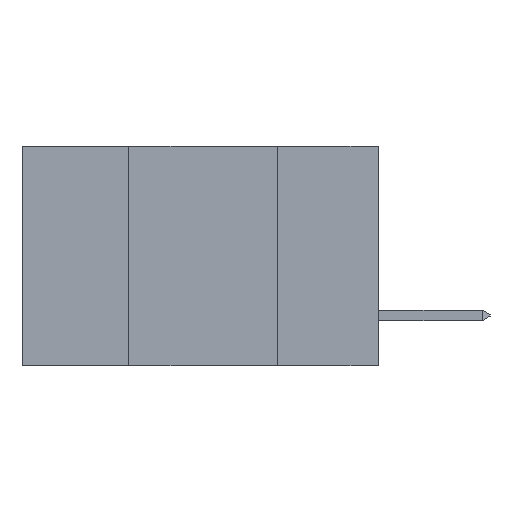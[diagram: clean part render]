
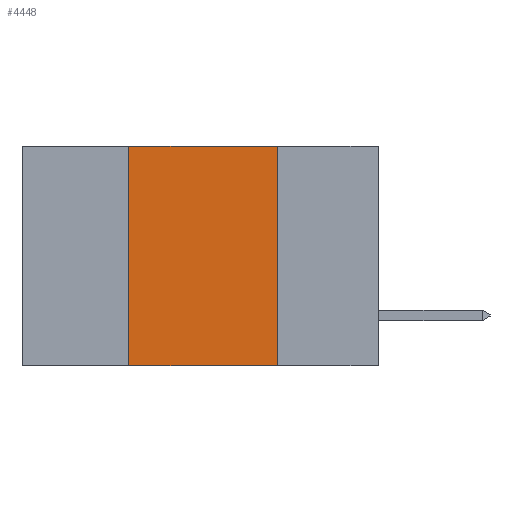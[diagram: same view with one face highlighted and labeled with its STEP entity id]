
A CAD part, left-side view. The second image highlights one B-rep face of the part: STEP entity #4448.
In plain terms, the highlighted planar face has unit normal (-1, 0, 0).
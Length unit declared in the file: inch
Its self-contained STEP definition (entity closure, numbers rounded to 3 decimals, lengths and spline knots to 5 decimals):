
#2800 = VERTEX_POINT ( 'NONE', #9452 ) ;
#3032 = DIRECTION ( 'NONE',  ( 0., 0., -1. ) ) ;
#3098 = DIRECTION ( 'NONE',  ( 1., 0., 0. ) ) ;
#4194 = VECTOR ( 'NONE', #26800, 39.37008 ) ;
#4448 = ADVANCED_FACE ( 'NONE', ( #22939 ), #6076, .F. ) ;
#4514 = CARTESIAN_POINT ( 'NONE',  ( 0., 0.17, 0. ) ) ;
#4547 = EDGE_CURVE ( 'NONE', #25164, #24724, #20202, .T. ) ;
#5257 = CARTESIAN_POINT ( 'NONE',  ( 0., 0.6, 0. ) ) ;
#6076 = PLANE ( 'NONE',  #16238 ) ;
#9062 = CARTESIAN_POINT ( 'NONE',  ( 0., 0.6, -0.37 ) ) ;
#9239 = EDGE_LOOP ( 'NONE', ( #10128, #17711, #11962, #24147 ) ) ;
#9452 = CARTESIAN_POINT ( 'NONE',  ( 0., 0.42, 0. ) ) ;
#9957 = VECTOR ( 'NONE', #14815, 39.37008 ) ;
#10106 = EDGE_CURVE ( 'NONE', #20956, #24724, #22826, .T. ) ;
#10128 = ORIENTED_EDGE ( 'NONE', *, *, #4547, .F. ) ;
#11547 = CARTESIAN_POINT ( 'NONE',  ( 0., 0.42, -0.37 ) ) ;
#11705 = EDGE_CURVE ( 'NONE', #2800, #25164, #14842, .T. ) ;
#11962 = ORIENTED_EDGE ( 'NONE', *, *, #20606, .F. ) ;
#12812 = CARTESIAN_POINT ( 'NONE',  ( 0., 0.42, 0. ) ) ;
#13532 = VECTOR ( 'NONE', #24804, 39.37008 ) ;
#14151 = CARTESIAN_POINT ( 'NONE',  ( 0., 0.6, 0. ) ) ;
#14815 = DIRECTION ( 'NONE',  ( 0., 0., 1. ) ) ;
#14842 = LINE ( 'NONE', #5257, #26573 ) ;
#15214 = LINE ( 'NONE', #12812, #9957 ) ;
#15602 = CARTESIAN_POINT ( 'NONE',  ( 0., 0.17, -0.37 ) ) ;
#16238 = AXIS2_PLACEMENT_3D ( 'NONE', #14151, #3098, #3032 ) ;
#17711 = ORIENTED_EDGE ( 'NONE', *, *, #11705, .F. ) ;
#20202 = LINE ( 'NONE', #4514, #13532 ) ;
#20606 = EDGE_CURVE ( 'NONE', #20956, #2800, #15214, .T. ) ;
#20956 = VERTEX_POINT ( 'NONE', #11547 ) ;
#21003 = DIRECTION ( 'NONE',  ( 0., -1., 0. ) ) ;
#22826 = LINE ( 'NONE', #9062, #4194 ) ;
#22939 = FACE_OUTER_BOUND ( 'NONE', #9239, .T. ) ;
#24147 = ORIENTED_EDGE ( 'NONE', *, *, #10106, .T. ) ;
#24724 = VERTEX_POINT ( 'NONE', #15602 ) ;
#24804 = DIRECTION ( 'NONE',  ( 0., 0., -1. ) ) ;
#25164 = VERTEX_POINT ( 'NONE', #26942 ) ;
#26573 = VECTOR ( 'NONE', #21003, 39.37008 ) ;
#26800 = DIRECTION ( 'NONE',  ( 0., -1., 0. ) ) ;
#26942 = CARTESIAN_POINT ( 'NONE',  ( 0., 0.17, 0. ) ) ;
